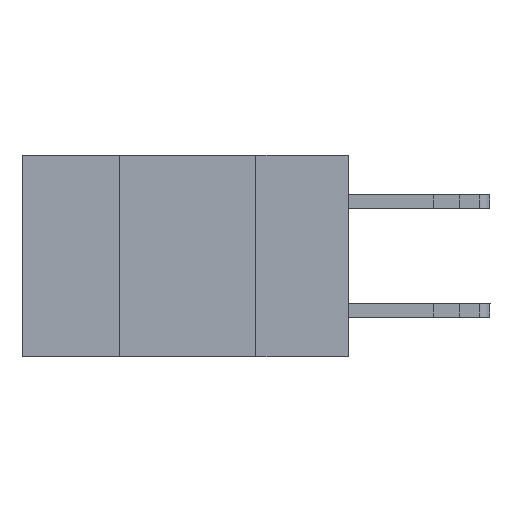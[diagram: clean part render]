
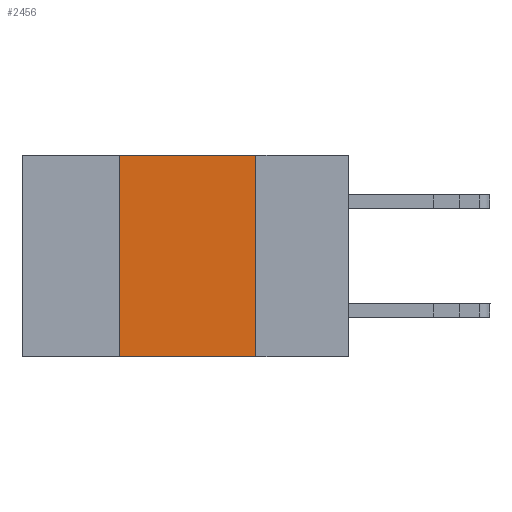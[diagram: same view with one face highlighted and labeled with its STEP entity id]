
A CAD part, left-side view. The second image highlights one B-rep face of the part: STEP entity #2456.
In plain terms, the highlighted planar face has unit normal (-1, 0, 0).
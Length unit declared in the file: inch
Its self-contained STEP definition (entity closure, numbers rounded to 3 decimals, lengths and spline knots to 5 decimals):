
#140 = EDGE_CURVE ( 'NONE', #3467, #5907, #8420, .T. ) ;
#555 = EDGE_LOOP ( 'NONE', ( #10100, #8149, #8626, #1535 ) ) ;
#801 = VECTOR ( 'NONE', #4562, 39.37008 ) ;
#1535 = ORIENTED_EDGE ( 'NONE', *, *, #2733, .T. ) ;
#1571 = CARTESIAN_POINT ( 'NONE',  ( 0., 0.42, 0. ) ) ;
#1705 = DIRECTION ( 'NONE',  ( 0., -1., 0. ) ) ;
#2456 = ADVANCED_FACE ( 'NONE', ( #8029 ), #7539, .F. ) ;
#2733 = EDGE_CURVE ( 'NONE', #3467, #11471, #2761, .T. ) ;
#2761 = LINE ( 'NONE', #4610, #801 ) ;
#3467 = VERTEX_POINT ( 'NONE', #11343 ) ;
#4562 = DIRECTION ( 'NONE',  ( 0., -1., 0. ) ) ;
#4610 = CARTESIAN_POINT ( 'NONE',  ( 0., 0.6, -0.37 ) ) ;
#5832 = VECTOR ( 'NONE', #7479, 39.37008 ) ;
#5907 = VERTEX_POINT ( 'NONE', #1571 ) ;
#6345 = DIRECTION ( 'NONE',  ( 0., 0., -1. ) ) ;
#6726 = VERTEX_POINT ( 'NONE', #11104 ) ;
#7353 = LINE ( 'NONE', #10307, #10488 ) ;
#7473 = DIRECTION ( 'NONE',  ( 0., 0., -1. ) ) ;
#7479 = DIRECTION ( 'NONE',  ( 0., 0., 1. ) ) ;
#7486 = DIRECTION ( 'NONE',  ( 1., 0., 0. ) ) ;
#7539 = PLANE ( 'NONE',  #10773 ) ;
#7724 = CARTESIAN_POINT ( 'NONE',  ( 0., 0.6, 0. ) ) ;
#7826 = CARTESIAN_POINT ( 'NONE',  ( 0., 0.42, -0.37 ) ) ;
#8029 = FACE_OUTER_BOUND ( 'NONE', #555, .T. ) ;
#8149 = ORIENTED_EDGE ( 'NONE', *, *, #11324, .F. ) ;
#8420 = LINE ( 'NONE', #7826, #5832 ) ;
#8553 = CARTESIAN_POINT ( 'NONE',  ( 0., 0.17, -0.37 ) ) ;
#8626 = ORIENTED_EDGE ( 'NONE', *, *, #140, .F. ) ;
#9199 = LINE ( 'NONE', #12014, #12207 ) ;
#10100 = ORIENTED_EDGE ( 'NONE', *, *, #10691, .F. ) ;
#10307 = CARTESIAN_POINT ( 'NONE',  ( 0., 0.6, 0. ) ) ;
#10488 = VECTOR ( 'NONE', #1705, 39.37008 ) ;
#10691 = EDGE_CURVE ( 'NONE', #6726, #11471, #9199, .T. ) ;
#10773 = AXIS2_PLACEMENT_3D ( 'NONE', #7724, #7486, #7473 ) ;
#11104 = CARTESIAN_POINT ( 'NONE',  ( 0., 0.17, 0. ) ) ;
#11324 = EDGE_CURVE ( 'NONE', #5907, #6726, #7353, .T. ) ;
#11343 = CARTESIAN_POINT ( 'NONE',  ( 0., 0.42, -0.37 ) ) ;
#11471 = VERTEX_POINT ( 'NONE', #8553 ) ;
#12014 = CARTESIAN_POINT ( 'NONE',  ( 0., 0.17, -0.37 ) ) ;
#12207 = VECTOR ( 'NONE', #6345, 39.37008 ) ;
